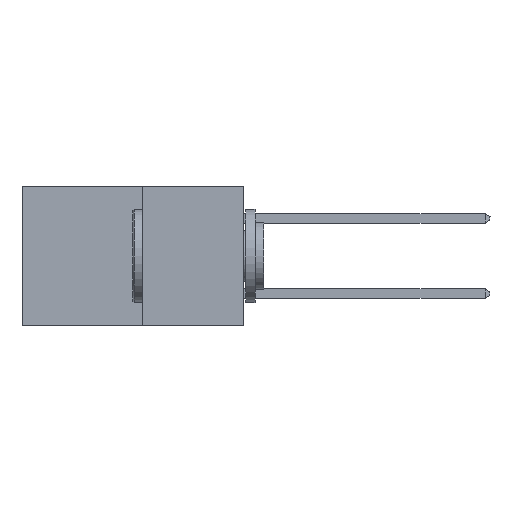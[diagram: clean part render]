
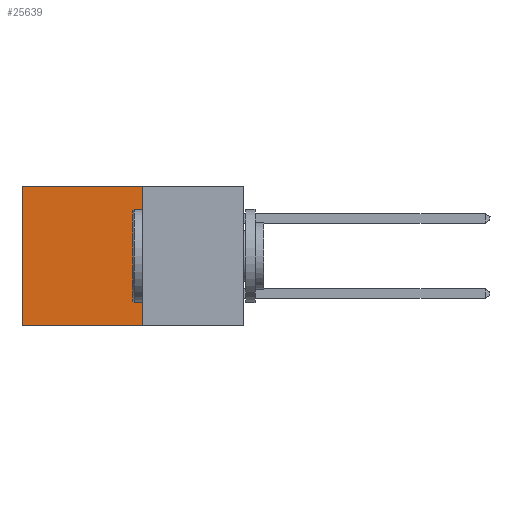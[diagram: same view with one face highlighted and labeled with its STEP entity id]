
A CAD part, left-side view. The second image highlights one B-rep face of the part: STEP entity #25639.
In plain terms, the highlighted planar face has unit normal (-1, 0, 0).
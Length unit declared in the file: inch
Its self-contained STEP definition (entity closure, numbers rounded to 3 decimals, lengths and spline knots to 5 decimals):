
#1046 = PLANE ( 'NONE',  #8045 ) ;
#2133 = DIRECTION ( 'NONE',  ( 0., 1., 0. ) ) ;
#2237 = CARTESIAN_POINT ( 'NONE',  ( 0.277, 0.59, 0. ) ) ;
#2811 = LINE ( 'NONE', #9045, #22423 ) ;
#3725 = DIRECTION ( 'NONE',  ( 0., 0., -1. ) ) ;
#4187 = ORIENTED_EDGE ( 'NONE', *, *, #31438, .F. ) ;
#6591 = FACE_OUTER_BOUND ( 'NONE', #32388, .T. ) ;
#6762 = VECTOR ( 'NONE', #19755, 39.37008 ) ;
#7597 = LINE ( 'NONE', #9107, #6762 ) ;
#7948 = EDGE_CURVE ( 'NONE', #22386, #17183, #29326, .T. ) ;
#8045 = AXIS2_PLACEMENT_3D ( 'NONE', #30112, #19748, #3725 ) ;
#9045 = CARTESIAN_POINT ( 'NONE',  ( 0.277, 0.27, 0. ) ) ;
#9107 = CARTESIAN_POINT ( 'NONE',  ( 0.277, 0.27, -0.37 ) ) ;
#9139 = ORIENTED_EDGE ( 'NONE', *, *, #34090, .T. ) ;
#11403 = ORIENTED_EDGE ( 'NONE', *, *, #7948, .T. ) ;
#11511 = EDGE_CURVE ( 'NONE', #31881, #17183, #29996, .T. ) ;
#12392 = ORIENTED_EDGE ( 'NONE', *, *, #11511, .F. ) ;
#17095 = DIRECTION ( 'NONE',  ( 0., 1., 0. ) ) ;
#17183 = VERTEX_POINT ( 'NONE', #33589 ) ;
#17692 = VECTOR ( 'NONE', #2133, 39.37008 ) ;
#18856 = CARTESIAN_POINT ( 'NONE',  ( 0.277, 0.59, -0.37 ) ) ;
#19748 = DIRECTION ( 'NONE',  ( 1., 0., 0. ) ) ;
#19755 = DIRECTION ( 'NONE',  ( 0., 0., -1. ) ) ;
#20817 = CARTESIAN_POINT ( 'NONE',  ( 0.277, 0.27, -0.37 ) ) ;
#22386 = VERTEX_POINT ( 'NONE', #2237 ) ;
#22423 = VECTOR ( 'NONE', #17095, 39.37008 ) ;
#22427 = VECTOR ( 'NONE', #26746, 39.37008 ) ;
#24052 = CARTESIAN_POINT ( 'NONE',  ( 0.277, 0.27, -0.37 ) ) ;
#25639 = ADVANCED_FACE ( 'NONE', ( #6591 ), #1046, .F. ) ;
#26746 = DIRECTION ( 'NONE',  ( 0., 0., -1. ) ) ;
#29066 = VERTEX_POINT ( 'NONE', #33725 ) ;
#29326 = LINE ( 'NONE', #18856, #22427 ) ;
#29996 = LINE ( 'NONE', #20817, #17692 ) ;
#30112 = CARTESIAN_POINT ( 'NONE',  ( 0.277, 0.27, -0.37 ) ) ;
#31438 = EDGE_CURVE ( 'NONE', #29066, #31881, #7597, .T. ) ;
#31881 = VERTEX_POINT ( 'NONE', #24052 ) ;
#32388 = EDGE_LOOP ( 'NONE', ( #11403, #12392, #4187, #9139 ) ) ;
#33589 = CARTESIAN_POINT ( 'NONE',  ( 0.277, 0.59, -0.37 ) ) ;
#33725 = CARTESIAN_POINT ( 'NONE',  ( 0.277, 0.27, 0. ) ) ;
#34090 = EDGE_CURVE ( 'NONE', #29066, #22386, #2811, .T. ) ;
